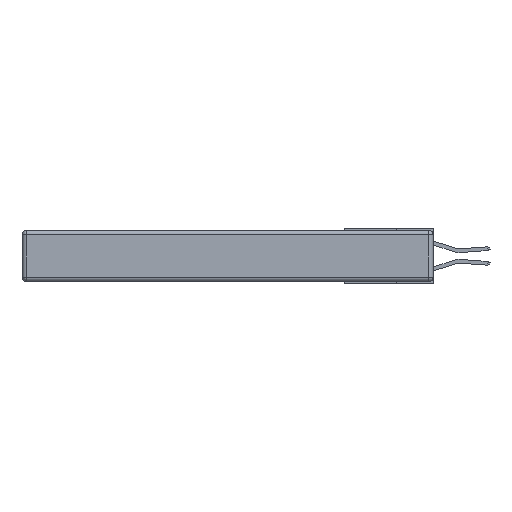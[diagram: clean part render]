
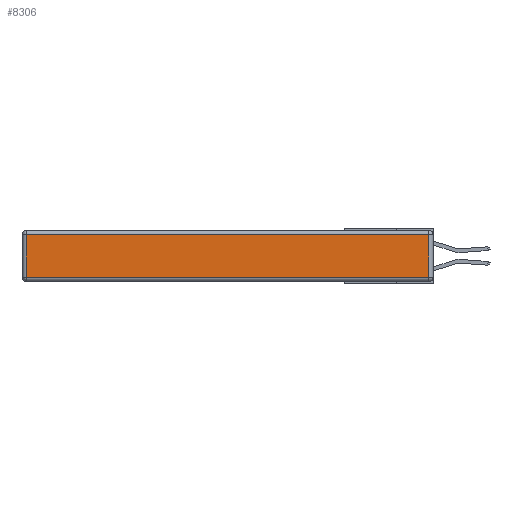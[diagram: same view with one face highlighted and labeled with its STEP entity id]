
A CAD part, left-side view. The second image highlights one B-rep face of the part: STEP entity #8306.
In plain terms, the highlighted planar face has unit normal (-1, 0, 0).
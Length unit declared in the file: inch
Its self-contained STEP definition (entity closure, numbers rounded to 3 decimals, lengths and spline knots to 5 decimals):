
#551 = VECTOR ( 'NONE', #2415, 39.37008 ) ;
#603 = ORIENTED_EDGE ( 'NONE', *, *, #25417, .T. ) ;
#791 = DIRECTION ( 'NONE',  ( 0., 1., 0. ) ) ;
#1012 = VECTOR ( 'NONE', #28743, 39.37008 ) ;
#1244 = ORIENTED_EDGE ( 'NONE', *, *, #9904, .T. ) ;
#2415 = DIRECTION ( 'NONE',  ( 0., 0., -1. ) ) ;
#3815 = VECTOR ( 'NONE', #791, 39.37008 ) ;
#5404 = LINE ( 'NONE', #13438, #551 ) ;
#5831 = AXIS2_PLACEMENT_3D ( 'NONE', #25764, #11480, #23449 ) ;
#5928 = CARTESIAN_POINT ( 'NONE',  ( 0., 0.03, -0.343 ) ) ;
#7996 = FACE_OUTER_BOUND ( 'NONE', #27955, .T. ) ;
#8306 = ADVANCED_FACE ( 'NONE', ( #7996 ), #23346, .T. ) ;
#9904 = EDGE_CURVE ( 'NONE', #27490, #16591, #19776, .T. ) ;
#11480 = DIRECTION ( 'NONE',  ( -1., 0., 0. ) ) ;
#11901 = EDGE_CURVE ( 'NONE', #20434, #20158, #30888, .T. ) ;
#13438 = CARTESIAN_POINT ( 'NONE',  ( 0., 2.72, -0.343 ) ) ;
#13550 = VECTOR ( 'NONE', #17641, 39.37008 ) ;
#14037 = CARTESIAN_POINT ( 'NONE',  ( 0., 0.03, -0.03 ) ) ;
#14985 = EDGE_CURVE ( 'NONE', #16591, #20434, #5404, .T. ) ;
#15399 = LINE ( 'NONE', #5928, #13550 ) ;
#16591 = VERTEX_POINT ( 'NONE', #25415 ) ;
#17308 = CARTESIAN_POINT ( 'NONE',  ( 0., 2.75, -0.03 ) ) ;
#17641 = DIRECTION ( 'NONE',  ( 0., 0., 1. ) ) ;
#17841 = CARTESIAN_POINT ( 'NONE',  ( 0., 2.72, -0.313 ) ) ;
#19776 = LINE ( 'NONE', #17308, #3815 ) ;
#20158 = VERTEX_POINT ( 'NONE', #26364 ) ;
#20434 = VERTEX_POINT ( 'NONE', #17841 ) ;
#22695 = ORIENTED_EDGE ( 'NONE', *, *, #14985, .T. ) ;
#23346 = PLANE ( 'NONE',  #5831 ) ;
#23449 = DIRECTION ( 'NONE',  ( 0., 0., 1. ) ) ;
#24386 = ORIENTED_EDGE ( 'NONE', *, *, #11901, .T. ) ;
#25415 = CARTESIAN_POINT ( 'NONE',  ( 0., 2.72, -0.03 ) ) ;
#25417 = EDGE_CURVE ( 'NONE', #20158, #27490, #15399, .T. ) ;
#25764 = CARTESIAN_POINT ( 'NONE',  ( 0., 0., -0.343 ) ) ;
#26364 = CARTESIAN_POINT ( 'NONE',  ( 0., 0.03, -0.313 ) ) ;
#27490 = VERTEX_POINT ( 'NONE', #14037 ) ;
#27955 = EDGE_LOOP ( 'NONE', ( #24386, #603, #1244, #22695 ) ) ;
#28743 = DIRECTION ( 'NONE',  ( 0., -1., 0. ) ) ;
#30747 = CARTESIAN_POINT ( 'NONE',  ( 0., 0., -0.313 ) ) ;
#30888 = LINE ( 'NONE', #30747, #1012 ) ;
